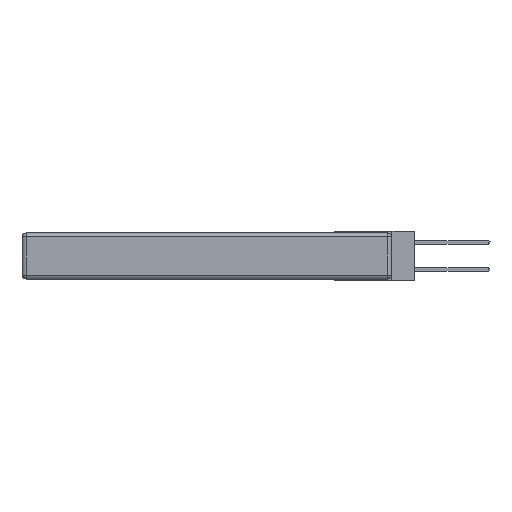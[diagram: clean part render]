
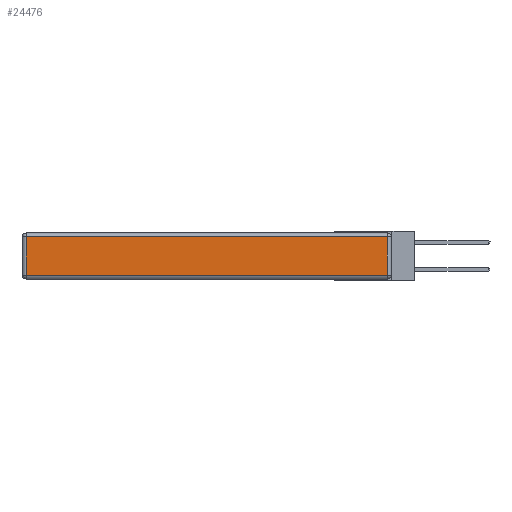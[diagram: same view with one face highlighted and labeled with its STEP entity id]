
A CAD part, left-side view. The second image highlights one B-rep face of the part: STEP entity #24476.
In plain terms, the highlighted planar face has unit normal (-1, 0, 0).
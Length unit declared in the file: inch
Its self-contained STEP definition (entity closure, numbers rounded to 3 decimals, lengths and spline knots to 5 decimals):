
#1693 = VERTEX_POINT ( 'NONE', #4354 ) ;
#2909 = EDGE_CURVE ( 'NONE', #1693, #14696, #19915, .T. ) ;
#4288 = VERTEX_POINT ( 'NONE', #17309 ) ;
#4354 = CARTESIAN_POINT ( 'NONE',  ( 0., 2.72, -0.03 ) ) ;
#8477 = DIRECTION ( 'NONE',  ( 0., 1., 0. ) ) ;
#8584 = CARTESIAN_POINT ( 'NONE',  ( 0., 0., -0.343 ) ) ;
#9268 = ORIENTED_EDGE ( 'NONE', *, *, #2909, .T. ) ;
#9360 = DIRECTION ( 'NONE',  ( 0., 0., 1. ) ) ;
#9489 = ORIENTED_EDGE ( 'NONE', *, *, #14970, .T. ) ;
#10654 = DIRECTION ( 'NONE',  ( 0., 0., 1. ) ) ;
#11573 = CARTESIAN_POINT ( 'NONE',  ( 0., 0., -0.313 ) ) ;
#11976 = VECTOR ( 'NONE', #15777, 39.37008 ) ;
#12288 = LINE ( 'NONE', #11573, #11976 ) ;
#12866 = CARTESIAN_POINT ( 'NONE',  ( 0., 2.75, -0.03 ) ) ;
#13279 = FACE_OUTER_BOUND ( 'NONE', #25227, .T. ) ;
#13602 = LINE ( 'NONE', #12866, #18418 ) ;
#14696 = VERTEX_POINT ( 'NONE', #18447 ) ;
#14970 = EDGE_CURVE ( 'NONE', #4288, #25592, #26306, .T. ) ;
#15775 = VECTOR ( 'NONE', #17418, 39.37008 ) ;
#15777 = DIRECTION ( 'NONE',  ( 0., -1., 0. ) ) ;
#17309 = CARTESIAN_POINT ( 'NONE',  ( 0., 0.03, -0.313 ) ) ;
#17418 = DIRECTION ( 'NONE',  ( 0., 0., -1. ) ) ;
#18418 = VECTOR ( 'NONE', #8477, 39.37008 ) ;
#18447 = CARTESIAN_POINT ( 'NONE',  ( 0., 2.72, -0.313 ) ) ;
#18997 = PLANE ( 'NONE',  #19933 ) ;
#19417 = CARTESIAN_POINT ( 'NONE',  ( 0., 0.03, -0.343 ) ) ;
#19553 = ORIENTED_EDGE ( 'NONE', *, *, #20036, .T. ) ;
#19915 = LINE ( 'NONE', #25523, #15775 ) ;
#19933 = AXIS2_PLACEMENT_3D ( 'NONE', #8584, #22899, #10654 ) ;
#20036 = EDGE_CURVE ( 'NONE', #25592, #1693, #13602, .T. ) ;
#22899 = DIRECTION ( 'NONE',  ( -1., 0., 0. ) ) ;
#22922 = ORIENTED_EDGE ( 'NONE', *, *, #25100, .T. ) ;
#23320 = CARTESIAN_POINT ( 'NONE',  ( 0., 0.03, -0.03 ) ) ;
#24476 = ADVANCED_FACE ( 'NONE', ( #13279 ), #18997, .T. ) ;
#25100 = EDGE_CURVE ( 'NONE', #14696, #4288, #12288, .T. ) ;
#25227 = EDGE_LOOP ( 'NONE', ( #22922, #9489, #19553, #9268 ) ) ;
#25523 = CARTESIAN_POINT ( 'NONE',  ( 0., 2.72, -0.343 ) ) ;
#25592 = VERTEX_POINT ( 'NONE', #23320 ) ;
#25681 = VECTOR ( 'NONE', #9360, 39.37008 ) ;
#26306 = LINE ( 'NONE', #19417, #25681 ) ;
